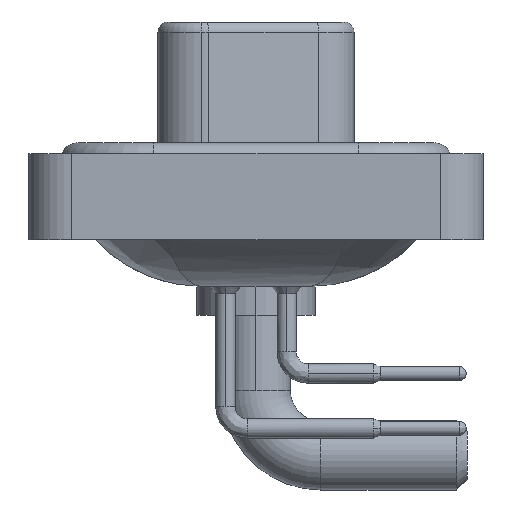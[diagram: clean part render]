
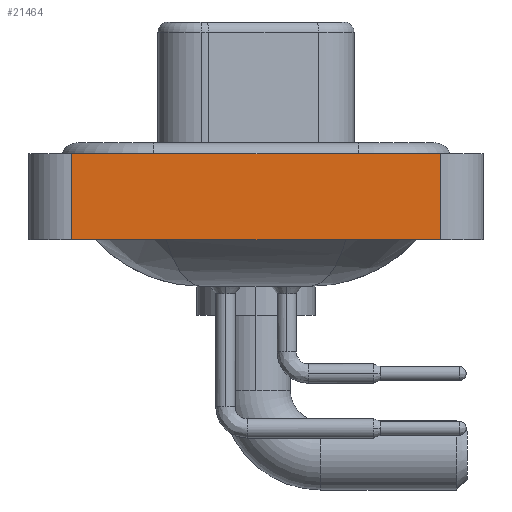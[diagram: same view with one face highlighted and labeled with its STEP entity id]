
A CAD part, left-side view. The second image highlights one B-rep face of the part: STEP entity #21464.
In plain terms, the highlighted planar face has unit normal (-1, 0, 0).
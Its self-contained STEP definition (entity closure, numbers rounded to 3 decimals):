
#858 = EDGE_CURVE ( 'NONE', #3992, #19990, #4938, .T. ) ;
#1088 = DIRECTION ( 'NONE',  ( 0., 0., 1. ) ) ;
#1184 = DIRECTION ( 'NONE',  ( 0., 0., 1. ) ) ;
#1229 = DIRECTION ( 'NONE',  ( 0., -1., 0. ) ) ;
#3992 = VERTEX_POINT ( 'NONE', #4677 ) ;
#4496 = VERTEX_POINT ( 'NONE', #20272 ) ;
#4677 = CARTESIAN_POINT ( 'NONE',  ( -7.25, 8.55, 0.4 ) ) ;
#4938 = LINE ( 'NONE', #8630, #21019 ) ;
#5023 = AXIS2_PLACEMENT_3D ( 'NONE', #19118, #22710, #1184 ) ;
#5456 = ORIENTED_EDGE ( 'NONE', *, *, #20850, .F. ) ;
#5869 = LINE ( 'NONE', #7708, #7770 ) ;
#5985 = DIRECTION ( 'NONE',  ( 0., 0., 1. ) ) ;
#6404 = PLANE ( 'NONE',  #5023 ) ;
#6869 = LINE ( 'NONE', #20997, #21272 ) ;
#7243 = LINE ( 'NONE', #9081, #8626 ) ;
#7708 = CARTESIAN_POINT ( 'NONE',  ( -7.25, -8.55, -3.6 ) ) ;
#7770 = VECTOR ( 'NONE', #5985, 1000. ) ;
#8626 = VECTOR ( 'NONE', #18006, 1000. ) ;
#8630 = CARTESIAN_POINT ( 'NONE',  ( -7.25, -8.55, 0.4 ) ) ;
#9081 = CARTESIAN_POINT ( 'NONE',  ( -7.25, -8.55, -3.6 ) ) ;
#9940 = EDGE_LOOP ( 'NONE', ( #18089, #22108, #5456, #18157 ) ) ;
#13446 = FACE_OUTER_BOUND ( 'NONE', #9940, .T. ) ;
#14572 = CARTESIAN_POINT ( 'NONE',  ( -7.25, -8.55, -3.6 ) ) ;
#16832 = EDGE_CURVE ( 'NONE', #22118, #19990, #5869, .T. ) ;
#18006 = DIRECTION ( 'NONE',  ( 0., -1., 0. ) ) ;
#18089 = ORIENTED_EDGE ( 'NONE', *, *, #16832, .T. ) ;
#18157 = ORIENTED_EDGE ( 'NONE', *, *, #20399, .T. ) ;
#19112 = CARTESIAN_POINT ( 'NONE',  ( -7.25, -8.55, 0.4 ) ) ;
#19118 = CARTESIAN_POINT ( 'NONE',  ( -7.25, -8.55, -3.6 ) ) ;
#19990 = VERTEX_POINT ( 'NONE', #19112 ) ;
#20272 = CARTESIAN_POINT ( 'NONE',  ( -7.25, 8.55, -3.6 ) ) ;
#20399 = EDGE_CURVE ( 'NONE', #4496, #22118, #7243, .T. ) ;
#20850 = EDGE_CURVE ( 'NONE', #4496, #3992, #6869, .T. ) ;
#20997 = CARTESIAN_POINT ( 'NONE',  ( -7.25, 8.55, -3.6 ) ) ;
#21019 = VECTOR ( 'NONE', #1229, 1000. ) ;
#21272 = VECTOR ( 'NONE', #1088, 1000. ) ;
#21464 = ADVANCED_FACE ( 'NONE', ( #13446 ), #6404, .T. ) ;
#22108 = ORIENTED_EDGE ( 'NONE', *, *, #858, .F. ) ;
#22118 = VERTEX_POINT ( 'NONE', #14572 ) ;
#22710 = DIRECTION ( 'NONE',  ( -1., 0., 0. ) ) ;
